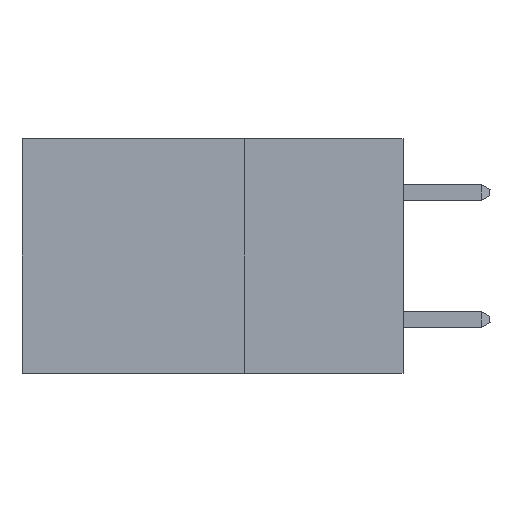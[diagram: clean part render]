
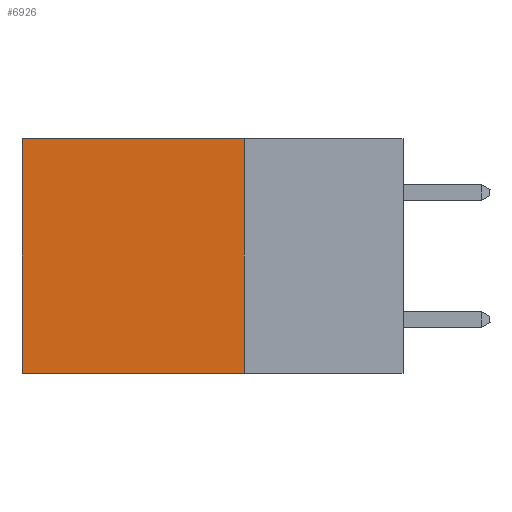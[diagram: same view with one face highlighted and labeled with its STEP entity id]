
A CAD part, left-side view. The second image highlights one B-rep face of the part: STEP entity #6926.
In plain terms, the highlighted planar face has unit normal (-1, 0, 0).
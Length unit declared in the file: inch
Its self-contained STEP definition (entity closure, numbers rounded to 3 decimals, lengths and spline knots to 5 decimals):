
#676 = LINE ( 'NONE', #25948, #37826 ) ;
#1638 = VERTEX_POINT ( 'NONE', #15169 ) ;
#2100 = AXIS2_PLACEMENT_3D ( 'NONE', #27324, #14018, #38843 ) ;
#3597 = LINE ( 'NONE', #24667, #38486 ) ;
#3629 = CARTESIAN_POINT ( 'NONE',  ( 0.2875, 0.25, 0. ) ) ;
#5160 = VERTEX_POINT ( 'NONE', #33393 ) ;
#5667 = VERTEX_POINT ( 'NONE', #7257 ) ;
#6375 = ORIENTED_EDGE ( 'NONE', *, *, #10872, .T. ) ;
#6926 = ADVANCED_FACE ( 'NONE', ( #28583 ), #23768, .F. ) ;
#7257 = CARTESIAN_POINT ( 'NONE',  ( 0.2875, 0.6, -0.37 ) ) ;
#9609 = EDGE_CURVE ( 'NONE', #1638, #5667, #3597, .T. ) ;
#10043 = DIRECTION ( 'NONE',  ( 0., 0., -1. ) ) ;
#10872 = EDGE_CURVE ( 'NONE', #26083, #1638, #22630, .T. ) ;
#14018 = DIRECTION ( 'NONE',  ( 1., 0., 0. ) ) ;
#15169 = CARTESIAN_POINT ( 'NONE',  ( 0.2875, 0.6, 0. ) ) ;
#19836 = VECTOR ( 'NONE', #27970, 39.37008 ) ;
#21848 = VECTOR ( 'NONE', #22795, 39.37008 ) ;
#22630 = LINE ( 'NONE', #38716, #19836 ) ;
#22795 = DIRECTION ( 'NONE',  ( 0., 1., 0. ) ) ;
#23768 = PLANE ( 'NONE',  #2100 ) ;
#24667 = CARTESIAN_POINT ( 'NONE',  ( 0.2875, 0.6, 0. ) ) ;
#25948 = CARTESIAN_POINT ( 'NONE',  ( 0.2875, 0.25, 0. ) ) ;
#26083 = VERTEX_POINT ( 'NONE', #3629 ) ;
#27324 = CARTESIAN_POINT ( 'NONE',  ( 0.2875, 0.25, 0. ) ) ;
#27970 = DIRECTION ( 'NONE',  ( 0., 1., 0. ) ) ;
#28583 = FACE_OUTER_BOUND ( 'NONE', #38926, .T. ) ;
#29843 = ORIENTED_EDGE ( 'NONE', *, *, #34922, .F. ) ;
#32618 = ORIENTED_EDGE ( 'NONE', *, *, #9609, .T. ) ;
#33393 = CARTESIAN_POINT ( 'NONE',  ( 0.2875, 0.25, -0.37 ) ) ;
#34922 = EDGE_CURVE ( 'NONE', #26083, #5160, #676, .T. ) ;
#37826 = VECTOR ( 'NONE', #40884, 39.37008 ) ;
#38486 = VECTOR ( 'NONE', #10043, 39.37008 ) ;
#38716 = CARTESIAN_POINT ( 'NONE',  ( 0.2875, 0.25, 0. ) ) ;
#38843 = DIRECTION ( 'NONE',  ( 0., 0., -1. ) ) ;
#38926 = EDGE_LOOP ( 'NONE', ( #32618, #46596, #29843, #6375 ) ) ;
#40721 = CARTESIAN_POINT ( 'NONE',  ( 0.2875, 0.25, -0.37 ) ) ;
#40884 = DIRECTION ( 'NONE',  ( 0., 0., -1. ) ) ;
#40983 = LINE ( 'NONE', #40721, #21848 ) ;
#44351 = EDGE_CURVE ( 'NONE', #5160, #5667, #40983, .T. ) ;
#46596 = ORIENTED_EDGE ( 'NONE', *, *, #44351, .F. ) ;
